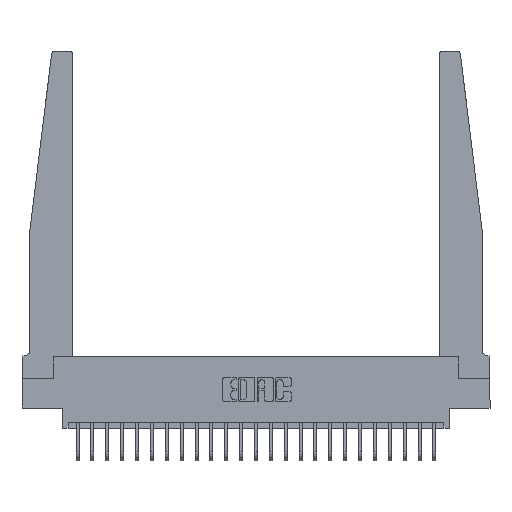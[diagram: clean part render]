
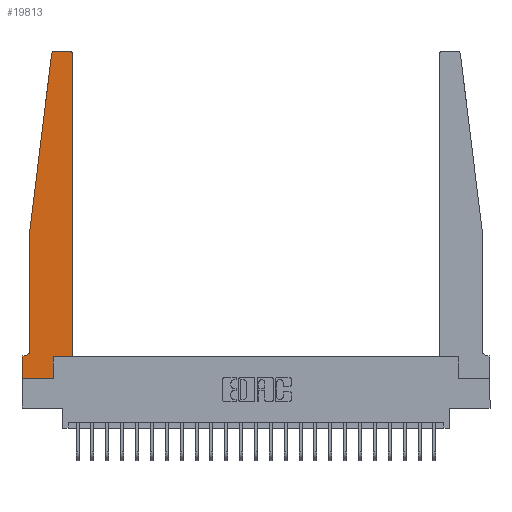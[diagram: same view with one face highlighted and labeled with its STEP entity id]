
A CAD part, top view. The second image highlights one B-rep face of the part: STEP entity #19813.
In plain terms, the highlighted planar face has unit normal (0, 0, 1).
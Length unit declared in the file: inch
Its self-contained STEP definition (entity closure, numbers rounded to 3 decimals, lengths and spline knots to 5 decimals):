
#594 = EDGE_CURVE ( 'NONE', #20300, #6946, #11691, .T. ) ;
#1015 = AXIS2_PLACEMENT_3D ( 'NONE', #14944, #2800, #8849 ) ;
#1050 = CIRCLE ( 'NONE', #8136, 0.03 ) ;
#1209 = CARTESIAN_POINT ( 'NONE',  ( 0.015, 0.1875, 0.37 ) ) ;
#1308 = CARTESIAN_POINT ( 'NONE',  ( 0.24675, 2.72367, 0.37 ) ) ;
#1501 = VECTOR ( 'NONE', #4784, 39.37008 ) ;
#2295 = ORIENTED_EDGE ( 'NONE', *, *, #20108, .T. ) ;
#2717 = EDGE_LOOP ( 'NONE', ( #16344, #5891, #18207, #23428, #10849, #25564, #16719, #2295, #21391, #25177, #3584, #23722 ) ) ;
#2800 = DIRECTION ( 'NONE',  ( 0., 0., 1. ) ) ;
#3199 = CARTESIAN_POINT ( 'NONE',  ( 0.425, 2.72, 0.37 ) ) ;
#3454 = CARTESIAN_POINT ( 'NONE',  ( 0.425, 0.18, 0.37 ) ) ;
#3584 = ORIENTED_EDGE ( 'NONE', *, *, #23469, .T. ) ;
#4010 = CARTESIAN_POINT ( 'NONE',  ( 0., 0.1875, 0.37 ) ) ;
#4132 = DIRECTION ( 'NONE',  ( 1., 0., 0. ) ) ;
#4316 = CARTESIAN_POINT ( 'NONE',  ( 0.395, 2.75, 0.37 ) ) ;
#4401 = VECTOR ( 'NONE', #4132, 39.37008 ) ;
#4784 = DIRECTION ( 'NONE',  ( 0., -1., 0. ) ) ;
#5198 = VERTEX_POINT ( 'NONE', #4010 ) ;
#5252 = EDGE_CURVE ( 'NONE', #14668, #18898, #7838, .T. ) ;
#5339 = EDGE_CURVE ( 'NONE', #17330, #14668, #12500, .T. ) ;
#5727 = DIRECTION ( 'NONE',  ( 1., 0., 0. ) ) ;
#5810 = EDGE_CURVE ( 'NONE', #6946, #22121, #13498, .T. ) ;
#5891 = ORIENTED_EDGE ( 'NONE', *, *, #5810, .T. ) ;
#6246 = CARTESIAN_POINT ( 'NONE',  ( 0.2605, 0.18, 0.37 ) ) ;
#6254 = CARTESIAN_POINT ( 'NONE',  ( 0.065, 1.25, 0.37 ) ) ;
#6613 = AXIS2_PLACEMENT_3D ( 'NONE', #8131, #24504, #18257 ) ;
#6742 = CARTESIAN_POINT ( 'NONE',  ( 0.27653, 2.75, 0.37 ) ) ;
#6802 = LINE ( 'NONE', #14489, #17571 ) ;
#6943 = VECTOR ( 'NONE', #14994, 39.37008 ) ;
#6946 = VERTEX_POINT ( 'NONE', #6742 ) ;
#7709 = CARTESIAN_POINT ( 'NONE',  ( 0.425, 0.18, 0.37 ) ) ;
#7804 = CARTESIAN_POINT ( 'NONE',  ( 0.2605, 0.18, 0.37 ) ) ;
#7838 = LINE ( 'NONE', #7709, #4401 ) ;
#7877 = EDGE_CURVE ( 'NONE', #14306, #5198, #15131, .T. ) ;
#7981 = CARTESIAN_POINT ( 'NONE',  ( 0.065, 1.25, 0.37 ) ) ;
#8131 = CARTESIAN_POINT ( 'NONE',  ( 0.015, 0.2375, 0.37 ) ) ;
#8136 = AXIS2_PLACEMENT_3D ( 'NONE', #21479, #25268, #9428 ) ;
#8148 = CARTESIAN_POINT ( 'NONE',  ( 0., 0., 0.37 ) ) ;
#8370 = DIRECTION ( 'NONE',  ( -0.122, -0.992, 0. ) ) ;
#8849 = DIRECTION ( 'NONE',  ( 1., 0., 0. ) ) ;
#9222 = CARTESIAN_POINT ( 'NONE',  ( 0., 0., 0.37 ) ) ;
#9228 = VECTOR ( 'NONE', #11800, 39.37008 ) ;
#9428 = DIRECTION ( 'NONE',  ( 1., 0., 0. ) ) ;
#9547 = PLANE ( 'NONE',  #22942 ) ;
#9959 = DIRECTION ( 'NONE',  ( 0., -1., 0. ) ) ;
#10237 = EDGE_CURVE ( 'NONE', #22121, #17878, #12391, .T. ) ;
#10849 = ORIENTED_EDGE ( 'NONE', *, *, #16328, .T. ) ;
#10997 = CARTESIAN_POINT ( 'NONE',  ( 0.065, 0.2375, 0.37 ) ) ;
#11691 = LINE ( 'NONE', #17292, #11886 ) ;
#11800 = DIRECTION ( 'NONE',  ( 1., 0., 0. ) ) ;
#11886 = VECTOR ( 'NONE', #17674, 39.37008 ) ;
#12248 = DIRECTION ( 'NONE',  ( 0., 1., 0. ) ) ;
#12391 = LINE ( 'NONE', #6254, #15652 ) ;
#12500 = LINE ( 'NONE', #6246, #16514 ) ;
#12701 = EDGE_CURVE ( 'NONE', #17878, #22145, #15677, .T. ) ;
#12798 = CARTESIAN_POINT ( 'NONE',  ( 0.065, 1.25, 0.37 ) ) ;
#13074 = EDGE_CURVE ( 'NONE', #15768, #20300, #1050, .T. ) ;
#13451 = EDGE_CURVE ( 'NONE', #5198, #25545, #16922, .T. ) ;
#13498 = CIRCLE ( 'NONE', #1015, 0.03 ) ;
#14306 = VERTEX_POINT ( 'NONE', #1209 ) ;
#14489 = CARTESIAN_POINT ( 'NONE',  ( 0.425, 0.18, 0.37 ) ) ;
#14668 = VERTEX_POINT ( 'NONE', #7804 ) ;
#14944 = CARTESIAN_POINT ( 'NONE',  ( 0.27653, 2.72, 0.37 ) ) ;
#14994 = DIRECTION ( 'NONE',  ( -1., 0., 0. ) ) ;
#15131 = LINE ( 'NONE', #17204, #6943 ) ;
#15636 = CARTESIAN_POINT ( 'NONE',  ( 0., 0.1875, 0.37 ) ) ;
#15652 = VECTOR ( 'NONE', #8370, 39.37008 ) ;
#15677 = LINE ( 'NONE', #7981, #18340 ) ;
#15716 = LINE ( 'NONE', #8148, #9228 ) ;
#15768 = VERTEX_POINT ( 'NONE', #3199 ) ;
#16325 = DIRECTION ( 'NONE',  ( 0., 1., 0. ) ) ;
#16328 = EDGE_CURVE ( 'NONE', #22145, #14306, #24060, .T. ) ;
#16344 = ORIENTED_EDGE ( 'NONE', *, *, #594, .T. ) ;
#16514 = VECTOR ( 'NONE', #12248, 39.37008 ) ;
#16719 = ORIENTED_EDGE ( 'NONE', *, *, #13451, .T. ) ;
#16922 = LINE ( 'NONE', #17045, #1501 ) ;
#17045 = CARTESIAN_POINT ( 'NONE',  ( 0., 0., 0.37 ) ) ;
#17204 = CARTESIAN_POINT ( 'NONE',  ( 0.065, 0.1875, 0.37 ) ) ;
#17292 = CARTESIAN_POINT ( 'NONE',  ( 0.25, 2.75, 0.37 ) ) ;
#17330 = VERTEX_POINT ( 'NONE', #17826 ) ;
#17571 = VECTOR ( 'NONE', #16325, 39.37008 ) ;
#17674 = DIRECTION ( 'NONE',  ( -1., 0., 0. ) ) ;
#17826 = CARTESIAN_POINT ( 'NONE',  ( 0.2605, 0., 0.37 ) ) ;
#17878 = VERTEX_POINT ( 'NONE', #12798 ) ;
#18207 = ORIENTED_EDGE ( 'NONE', *, *, #10237, .T. ) ;
#18257 = DIRECTION ( 'NONE',  ( -1., 0., 0. ) ) ;
#18340 = VECTOR ( 'NONE', #9959, 39.37008 ) ;
#18898 = VERTEX_POINT ( 'NONE', #3454 ) ;
#19813 = ADVANCED_FACE ( 'NONE', ( #25505 ), #9547, .T. ) ;
#20108 = EDGE_CURVE ( 'NONE', #25545, #17330, #15716, .T. ) ;
#20300 = VERTEX_POINT ( 'NONE', #4316 ) ;
#21391 = ORIENTED_EDGE ( 'NONE', *, *, #5339, .T. ) ;
#21479 = CARTESIAN_POINT ( 'NONE',  ( 0.395, 2.72, 0.37 ) ) ;
#22121 = VERTEX_POINT ( 'NONE', #1308 ) ;
#22145 = VERTEX_POINT ( 'NONE', #10997 ) ;
#22942 = AXIS2_PLACEMENT_3D ( 'NONE', #15636, #23557, #5727 ) ;
#23428 = ORIENTED_EDGE ( 'NONE', *, *, #12701, .T. ) ;
#23469 = EDGE_CURVE ( 'NONE', #18898, #15768, #6802, .T. ) ;
#23557 = DIRECTION ( 'NONE',  ( 0., 0., 1. ) ) ;
#23722 = ORIENTED_EDGE ( 'NONE', *, *, #13074, .T. ) ;
#24060 = CIRCLE ( 'NONE', #6613, 0.05 ) ;
#24504 = DIRECTION ( 'NONE',  ( 0., 0., -1. ) ) ;
#25177 = ORIENTED_EDGE ( 'NONE', *, *, #5252, .T. ) ;
#25268 = DIRECTION ( 'NONE',  ( 0., 0., 1. ) ) ;
#25505 = FACE_OUTER_BOUND ( 'NONE', #2717, .T. ) ;
#25545 = VERTEX_POINT ( 'NONE', #9222 ) ;
#25564 = ORIENTED_EDGE ( 'NONE', *, *, #7877, .T. ) ;
